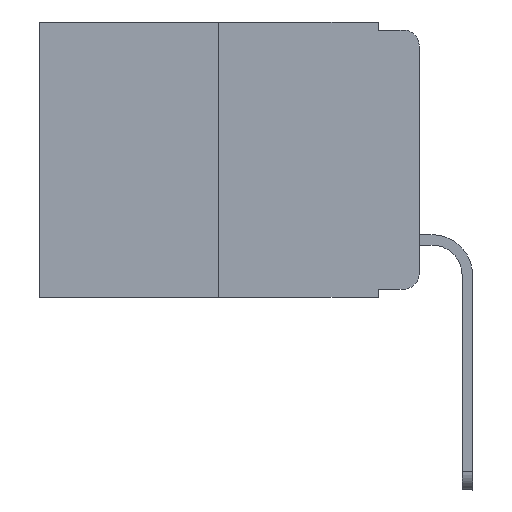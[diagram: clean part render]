
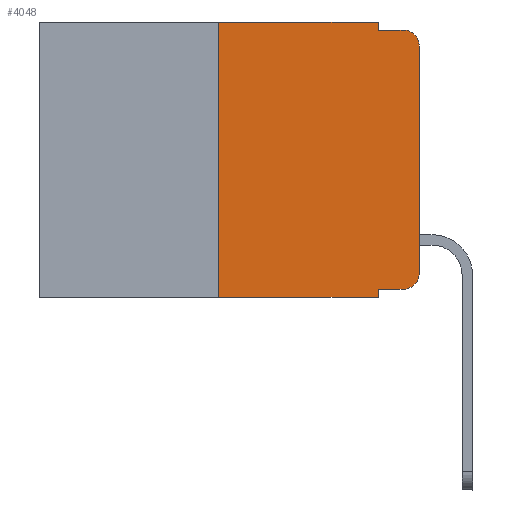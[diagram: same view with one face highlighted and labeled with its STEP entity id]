
A CAD part, left-side view. The second image highlights one B-rep face of the part: STEP entity #4048.
In plain terms, the highlighted planar face has unit normal (-1, 0, 0).
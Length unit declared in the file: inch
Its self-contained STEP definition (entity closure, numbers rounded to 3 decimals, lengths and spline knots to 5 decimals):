
#564 = CARTESIAN_POINT ( 'NONE',  ( 0., 0., -0.313 ) ) ;
#826 = VERTEX_POINT ( 'NONE', #17432 ) ;
#860 = CARTESIAN_POINT ( 'NONE',  ( 0., 0.473, 0. ) ) ;
#861 = ORIENTED_EDGE ( 'NONE', *, *, #7682, .T. ) ;
#1007 = LINE ( 'NONE', #4208, #16109 ) ;
#1043 = ORIENTED_EDGE ( 'NONE', *, *, #10302, .T. ) ;
#1108 = EDGE_CURVE ( 'NONE', #16806, #826, #1007, .T. ) ;
#1230 = CARTESIAN_POINT ( 'NONE',  ( 0., 0.473, -0.343 ) ) ;
#1326 = DIRECTION ( 'NONE',  ( 0., -1., 0. ) ) ;
#1619 = DIRECTION ( 'NONE',  ( 0., -1., 0. ) ) ;
#1838 = AXIS2_PLACEMENT_3D ( 'NONE', #17884, #19236, #1879 ) ;
#1879 = DIRECTION ( 'NONE',  ( 0., 0., -1. ) ) ;
#2328 = ORIENTED_EDGE ( 'NONE', *, *, #10934, .F. ) ;
#2513 = VECTOR ( 'NONE', #19010, 39.37008 ) ;
#3288 = ORIENTED_EDGE ( 'NONE', *, *, #13149, .F. ) ;
#3309 = CARTESIAN_POINT ( 'NONE',  ( 0., 0., 0. ) ) ;
#3378 = VECTOR ( 'NONE', #19003, 39.37008 ) ;
#3407 = LINE ( 'NONE', #3309, #3378 ) ;
#3693 = CARTESIAN_POINT ( 'NONE',  ( 0., 0.051, 0. ) ) ;
#3988 = ORIENTED_EDGE ( 'NONE', *, *, #9753, .T. ) ;
#4048 = ADVANCED_FACE ( 'NONE', ( #14902 ), #15000, .F. ) ;
#4208 = CARTESIAN_POINT ( 'NONE',  ( 0., 0.25, 0. ) ) ;
#4307 = CARTESIAN_POINT ( 'NONE',  ( 0., 0.051, -0.343 ) ) ;
#4382 = LINE ( 'NONE', #20378, #17733 ) ;
#4605 = ORIENTED_EDGE ( 'NONE', *, *, #9441, .T. ) ;
#4639 = LINE ( 'NONE', #12375, #17171 ) ;
#5077 = DIRECTION ( 'NONE',  ( -1., 0., 0. ) ) ;
#5557 = DIRECTION ( 'NONE',  ( 0., 0., 1. ) ) ;
#5716 = DIRECTION ( 'NONE',  ( 1., 0., 0. ) ) ;
#5943 = EDGE_CURVE ( 'NONE', #14019, #20388, #11011, .T. ) ;
#6179 = DIRECTION ( 'NONE',  ( 0., -1., 0. ) ) ;
#6236 = DIRECTION ( 'NONE',  ( 0., -1., 0. ) ) ;
#6348 = CARTESIAN_POINT ( 'NONE',  ( 0., 0.02, -0.01 ) ) ;
#7030 = ORIENTED_EDGE ( 'NONE', *, *, #1108, .F. ) ;
#7146 = ORIENTED_EDGE ( 'NONE', *, *, #19763, .T. ) ;
#7167 = DIRECTION ( 'NONE',  ( 0., 0., -1. ) ) ;
#7257 = CARTESIAN_POINT ( 'NONE',  ( 0., 0.25, -0.343 ) ) ;
#7546 = CARTESIAN_POINT ( 'NONE',  ( 0., 0., -0.03 ) ) ;
#7682 = EDGE_CURVE ( 'NONE', #14892, #15006, #9177, .T. ) ;
#7685 = VECTOR ( 'NONE', #6179, 39.37008 ) ;
#8102 = CIRCLE ( 'NONE', #1838, 0.02 ) ;
#9177 = LINE ( 'NONE', #15462, #10051 ) ;
#9441 = EDGE_CURVE ( 'NONE', #11697, #18090, #3407, .T. ) ;
#9486 = CIRCLE ( 'NONE', #10794, 0.02 ) ;
#9586 = ORIENTED_EDGE ( 'NONE', *, *, #5943, .F. ) ;
#9753 = EDGE_CURVE ( 'NONE', #16806, #14617, #16903, .T. ) ;
#10051 = VECTOR ( 'NONE', #1326, 39.37008 ) ;
#10302 = EDGE_CURVE ( 'NONE', #18090, #20388, #8102, .T. ) ;
#10794 = AXIS2_PLACEMENT_3D ( 'NONE', #19226, #5077, #11365 ) ;
#10934 = EDGE_CURVE ( 'NONE', #14892, #14617, #4639, .T. ) ;
#11011 = LINE ( 'NONE', #17414, #11794 ) ;
#11365 = DIRECTION ( 'NONE',  ( 0., 0., -1. ) ) ;
#11697 = VERTEX_POINT ( 'NONE', #564 ) ;
#11794 = VECTOR ( 'NONE', #1619, 39.37008 ) ;
#12375 = CARTESIAN_POINT ( 'NONE',  ( 0., 0.051, 0. ) ) ;
#12713 = CARTESIAN_POINT ( 'NONE',  ( 0., 0.051, 0. ) ) ;
#13149 = EDGE_CURVE ( 'NONE', #826, #15771, #4382, .T. ) ;
#13557 = ORIENTED_EDGE ( 'NONE', *, *, #16934, .F. ) ;
#13571 = CARTESIAN_POINT ( 'NONE',  ( 0., 0.02, -0.333 ) ) ;
#14019 = VERTEX_POINT ( 'NONE', #14856 ) ;
#14617 = VERTEX_POINT ( 'NONE', #4307 ) ;
#14856 = CARTESIAN_POINT ( 'NONE',  ( 0., 0.051, -0.01 ) ) ;
#14892 = VERTEX_POINT ( 'NONE', #17808 ) ;
#14902 = FACE_OUTER_BOUND ( 'NONE', #15501, .T. ) ;
#15000 = PLANE ( 'NONE',  #18502 ) ;
#15006 = VERTEX_POINT ( 'NONE', #13571 ) ;
#15462 = CARTESIAN_POINT ( 'NONE',  ( 0., 0.051, -0.333 ) ) ;
#15475 = DIRECTION ( 'NONE',  ( 0., 0., -1. ) ) ;
#15501 = EDGE_LOOP ( 'NONE', ( #4605, #1043, #9586, #13557, #3288, #7030, #3988, #2328, #861, #7146 ) ) ;
#15771 = VERTEX_POINT ( 'NONE', #3693 ) ;
#16109 = VECTOR ( 'NONE', #5557, 39.37008 ) ;
#16806 = VERTEX_POINT ( 'NONE', #7257 ) ;
#16903 = LINE ( 'NONE', #1230, #7685 ) ;
#16934 = EDGE_CURVE ( 'NONE', #15771, #14019, #20352, .T. ) ;
#17171 = VECTOR ( 'NONE', #15475, 39.37008 ) ;
#17414 = CARTESIAN_POINT ( 'NONE',  ( 0., 0.051, -0.01 ) ) ;
#17432 = CARTESIAN_POINT ( 'NONE',  ( 0., 0.25, 0. ) ) ;
#17733 = VECTOR ( 'NONE', #6236, 39.37008 ) ;
#17808 = CARTESIAN_POINT ( 'NONE',  ( 0., 0.051, -0.333 ) ) ;
#17884 = CARTESIAN_POINT ( 'NONE',  ( 0., 0.02, -0.03 ) ) ;
#18090 = VERTEX_POINT ( 'NONE', #7546 ) ;
#18502 = AXIS2_PLACEMENT_3D ( 'NONE', #860, #5716, #7167 ) ;
#19003 = DIRECTION ( 'NONE',  ( 0., 0., 1. ) ) ;
#19010 = DIRECTION ( 'NONE',  ( 0., 0., -1. ) ) ;
#19226 = CARTESIAN_POINT ( 'NONE',  ( 0., 0.02, -0.313 ) ) ;
#19236 = DIRECTION ( 'NONE',  ( -1., 0., 0. ) ) ;
#19763 = EDGE_CURVE ( 'NONE', #15006, #11697, #9486, .T. ) ;
#20352 = LINE ( 'NONE', #12713, #2513 ) ;
#20378 = CARTESIAN_POINT ( 'NONE',  ( 0., 0.473, 0. ) ) ;
#20388 = VERTEX_POINT ( 'NONE', #6348 ) ;
